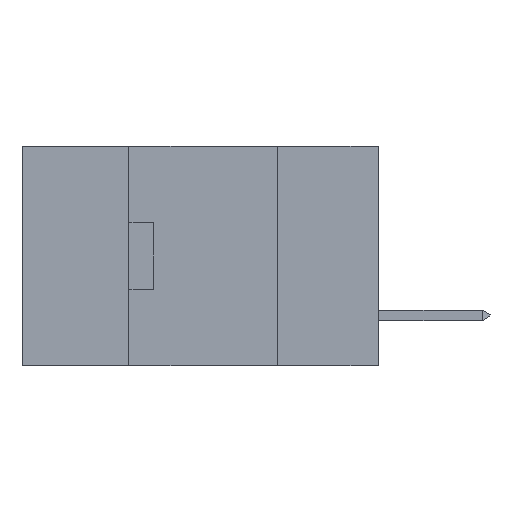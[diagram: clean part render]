
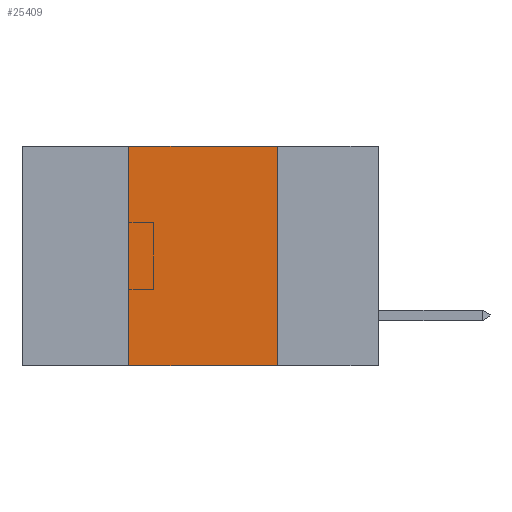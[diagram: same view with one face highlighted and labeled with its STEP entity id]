
A CAD part, left-side view. The second image highlights one B-rep face of the part: STEP entity #25409.
In plain terms, the highlighted planar face has unit normal (-1, 0, 0).
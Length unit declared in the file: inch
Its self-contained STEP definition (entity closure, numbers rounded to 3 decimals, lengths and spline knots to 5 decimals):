
#1546 = PLANE ( 'NONE',  #1757 ) ;
#1678 = FACE_OUTER_BOUND ( 'NONE', #8424, .T. ) ;
#1757 = AXIS2_PLACEMENT_3D ( 'NONE', #9809, #6150, #11956 ) ;
#5283 = LINE ( 'NONE', #21862, #12630 ) ;
#5528 = LINE ( 'NONE', #7175, #18110 ) ;
#6150 = DIRECTION ( 'NONE',  ( 1., 0., 0. ) ) ;
#7175 = CARTESIAN_POINT ( 'NONE',  ( 0., 0.6, -0.37 ) ) ;
#7239 = CARTESIAN_POINT ( 'NONE',  ( 0., 0.17, -0.37 ) ) ;
#7463 = CARTESIAN_POINT ( 'NONE',  ( 0., 0.42, 0. ) ) ;
#7501 = EDGE_CURVE ( 'NONE', #25663, #14211, #13031, .T. ) ;
#8424 = EDGE_LOOP ( 'NONE', ( #22043, #18172, #25437, #14538 ) ) ;
#9809 = CARTESIAN_POINT ( 'NONE',  ( 0., 0.6, 0. ) ) ;
#9877 = VECTOR ( 'NONE', #23635, 39.37008 ) ;
#11778 = DIRECTION ( 'NONE',  ( 0., 0., 1. ) ) ;
#11811 = VERTEX_POINT ( 'NONE', #12697 ) ;
#11956 = DIRECTION ( 'NONE',  ( 0., 0., -1. ) ) ;
#12630 = VECTOR ( 'NONE', #11778, 39.37008 ) ;
#12697 = CARTESIAN_POINT ( 'NONE',  ( 0., 0.42, -0.37 ) ) ;
#12981 = VERTEX_POINT ( 'NONE', #7463 ) ;
#13031 = LINE ( 'NONE', #7239, #24025 ) ;
#13136 = CARTESIAN_POINT ( 'NONE',  ( 0., 0.17, 0. ) ) ;
#13390 = LINE ( 'NONE', #26067, #9877 ) ;
#14211 = VERTEX_POINT ( 'NONE', #16682 ) ;
#14538 = ORIENTED_EDGE ( 'NONE', *, *, #24328, .T. ) ;
#16196 = EDGE_CURVE ( 'NONE', #11811, #12981, #5283, .T. ) ;
#16682 = CARTESIAN_POINT ( 'NONE',  ( 0., 0.17, -0.37 ) ) ;
#18110 = VECTOR ( 'NONE', #26037, 39.37008 ) ;
#18172 = ORIENTED_EDGE ( 'NONE', *, *, #22641, .F. ) ;
#21245 = DIRECTION ( 'NONE',  ( 0., 0., -1. ) ) ;
#21862 = CARTESIAN_POINT ( 'NONE',  ( 0., 0.42, -0.37 ) ) ;
#22043 = ORIENTED_EDGE ( 'NONE', *, *, #7501, .F. ) ;
#22641 = EDGE_CURVE ( 'NONE', #12981, #25663, #13390, .T. ) ;
#23635 = DIRECTION ( 'NONE',  ( 0., -1., 0. ) ) ;
#24025 = VECTOR ( 'NONE', #21245, 39.37008 ) ;
#24328 = EDGE_CURVE ( 'NONE', #11811, #14211, #5528, .T. ) ;
#25409 = ADVANCED_FACE ( 'NONE', ( #1678 ), #1546, .F. ) ;
#25437 = ORIENTED_EDGE ( 'NONE', *, *, #16196, .F. ) ;
#25663 = VERTEX_POINT ( 'NONE', #13136 ) ;
#26037 = DIRECTION ( 'NONE',  ( 0., -1., 0. ) ) ;
#26067 = CARTESIAN_POINT ( 'NONE',  ( 0., 0.6, 0. ) ) ;
